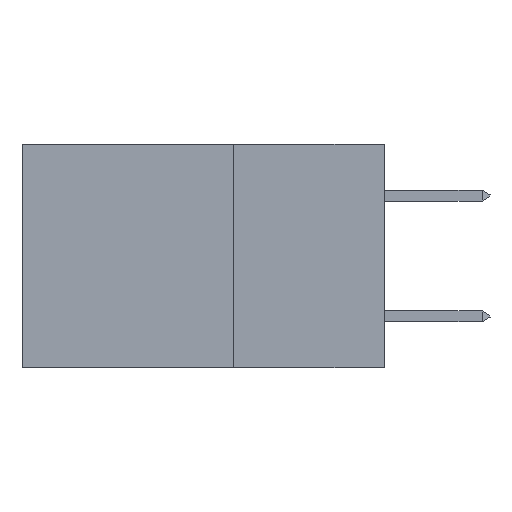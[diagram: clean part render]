
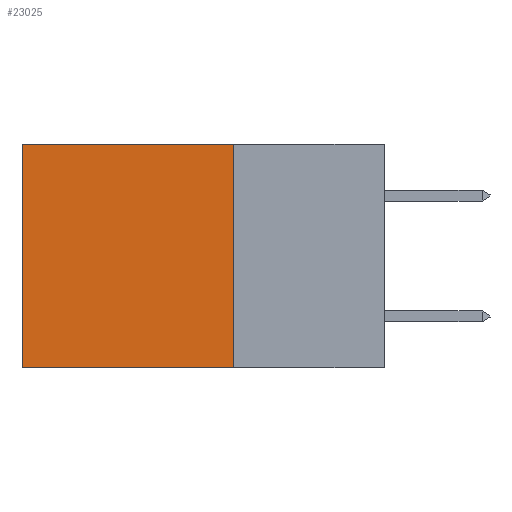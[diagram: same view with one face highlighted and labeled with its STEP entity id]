
A CAD part, left-side view. The second image highlights one B-rep face of the part: STEP entity #23025.
In plain terms, the highlighted planar face has unit normal (-1, 0, 0).
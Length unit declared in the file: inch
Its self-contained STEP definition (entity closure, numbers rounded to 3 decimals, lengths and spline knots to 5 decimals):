
#320 = EDGE_LOOP ( 'NONE', ( #5380, #29324, #21290, #25228 ) ) ;
#492 = EDGE_CURVE ( 'NONE', #1192, #24034, #16865, .T. ) ;
#656 = EDGE_CURVE ( 'NONE', #18508, #24034, #12207, .T. ) ;
#1192 = VERTEX_POINT ( 'NONE', #7794 ) ;
#3046 = DIRECTION ( 'NONE',  ( 1., 0., 0. ) ) ;
#4920 = VECTOR ( 'NONE', #23791, 39.37008 ) ;
#5006 = VERTEX_POINT ( 'NONE', #16156 ) ;
#5314 = CARTESIAN_POINT ( 'NONE',  ( 0.2875, 0.6, -0.37 ) ) ;
#5380 = ORIENTED_EDGE ( 'NONE', *, *, #656, .T. ) ;
#7794 = CARTESIAN_POINT ( 'NONE',  ( 0.2875, 0.25, -0.37 ) ) ;
#9945 = CARTESIAN_POINT ( 'NONE',  ( 0.2875, 0.25, 0. ) ) ;
#11030 = LINE ( 'NONE', #13987, #25170 ) ;
#11788 = CARTESIAN_POINT ( 'NONE',  ( 0.2875, 0.25, -0.37 ) ) ;
#12207 = LINE ( 'NONE', #29122, #23295 ) ;
#12608 = CARTESIAN_POINT ( 'NONE',  ( 0.2875, 0.6, 0. ) ) ;
#12928 = AXIS2_PLACEMENT_3D ( 'NONE', #29867, #3046, #29668 ) ;
#13987 = CARTESIAN_POINT ( 'NONE',  ( 0.2875, 0.25, 0. ) ) ;
#14959 = PLANE ( 'NONE',  #12928 ) ;
#16156 = CARTESIAN_POINT ( 'NONE',  ( 0.2875, 0.25, 0. ) ) ;
#16865 = LINE ( 'NONE', #11788, #4920 ) ;
#18508 = VERTEX_POINT ( 'NONE', #12608 ) ;
#18889 = VECTOR ( 'NONE', #22077, 39.37008 ) ;
#20161 = DIRECTION ( 'NONE',  ( 0., 0., -1. ) ) ;
#21290 = ORIENTED_EDGE ( 'NONE', *, *, #29451, .F. ) ;
#22077 = DIRECTION ( 'NONE',  ( 0., 1., 0. ) ) ;
#22088 = FACE_OUTER_BOUND ( 'NONE', #320, .T. ) ;
#23025 = ADVANCED_FACE ( 'NONE', ( #22088 ), #14959, .F. ) ;
#23295 = VECTOR ( 'NONE', #20161, 39.37008 ) ;
#23791 = DIRECTION ( 'NONE',  ( 0., 1., 0. ) ) ;
#24034 = VERTEX_POINT ( 'NONE', #5314 ) ;
#25170 = VECTOR ( 'NONE', #30962, 39.37008 ) ;
#25228 = ORIENTED_EDGE ( 'NONE', *, *, #30328, .T. ) ;
#29122 = CARTESIAN_POINT ( 'NONE',  ( 0.2875, 0.6, 0. ) ) ;
#29324 = ORIENTED_EDGE ( 'NONE', *, *, #492, .F. ) ;
#29451 = EDGE_CURVE ( 'NONE', #5006, #1192, #11030, .T. ) ;
#29668 = DIRECTION ( 'NONE',  ( 0., 0., -1. ) ) ;
#29867 = CARTESIAN_POINT ( 'NONE',  ( 0.2875, 0.25, 0. ) ) ;
#30247 = LINE ( 'NONE', #9945, #18889 ) ;
#30328 = EDGE_CURVE ( 'NONE', #5006, #18508, #30247, .T. ) ;
#30962 = DIRECTION ( 'NONE',  ( 0., 0., -1. ) ) ;
